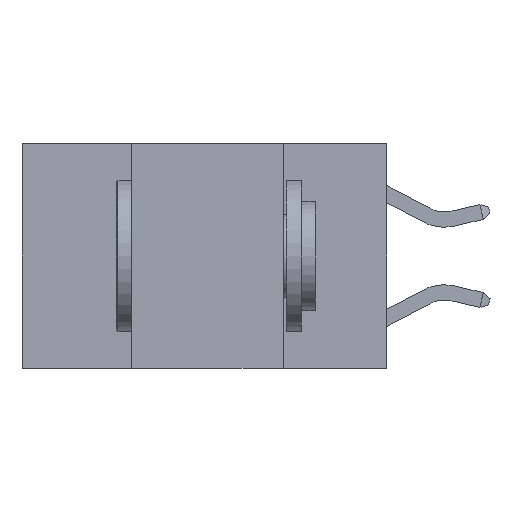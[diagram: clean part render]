
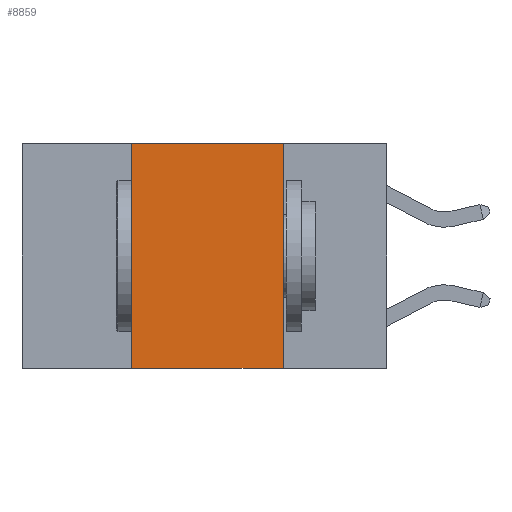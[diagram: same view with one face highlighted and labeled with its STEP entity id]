
A CAD part, left-side view. The second image highlights one B-rep face of the part: STEP entity #8859.
In plain terms, the highlighted planar face has unit normal (-1, 0, 0).
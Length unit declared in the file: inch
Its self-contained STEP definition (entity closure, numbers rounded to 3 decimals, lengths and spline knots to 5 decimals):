
#176 = VERTEX_POINT ( 'NONE', #12763 ) ;
#252 = PLANE ( 'NONE',  #11860 ) ;
#392 = CARTESIAN_POINT ( 'NONE',  ( 0., 0.6, 0. ) ) ;
#2381 = EDGE_CURVE ( 'NONE', #11145, #176, #7924, .T. ) ;
#2839 = FACE_OUTER_BOUND ( 'NONE', #3261, .T. ) ;
#3261 = EDGE_LOOP ( 'NONE', ( #10257, #10424, #11342, #3564 ) ) ;
#3564 = ORIENTED_EDGE ( 'NONE', *, *, #5597, .T. ) ;
#3608 = VERTEX_POINT ( 'NONE', #7484 ) ;
#3792 = VERTEX_POINT ( 'NONE', #4739 ) ;
#4494 = LINE ( 'NONE', #392, #9516 ) ;
#4739 = CARTESIAN_POINT ( 'NONE',  ( 0., 0.17, 0. ) ) ;
#5171 = CARTESIAN_POINT ( 'NONE',  ( 0., 0.17, 0. ) ) ;
#5269 = DIRECTION ( 'NONE',  ( 0., 0., -1. ) ) ;
#5597 = EDGE_CURVE ( 'NONE', #11145, #3608, #9882, .T. ) ;
#5792 = VECTOR ( 'NONE', #7195, 39.37008 ) ;
#5926 = EDGE_CURVE ( 'NONE', #3792, #3608, #8476, .T. ) ;
#6705 = CARTESIAN_POINT ( 'NONE',  ( 0., 0.6, -0.37 ) ) ;
#7195 = DIRECTION ( 'NONE',  ( 0., 0., -1. ) ) ;
#7484 = CARTESIAN_POINT ( 'NONE',  ( 0., 0.17, -0.37 ) ) ;
#7616 = VECTOR ( 'NONE', #11719, 39.37008 ) ;
#7924 = LINE ( 'NONE', #9748, #7616 ) ;
#8218 = CARTESIAN_POINT ( 'NONE',  ( 0., 0.6, 0. ) ) ;
#8476 = LINE ( 'NONE', #5171, #5792 ) ;
#8859 = ADVANCED_FACE ( 'NONE', ( #2839 ), #252, .F. ) ;
#9516 = VECTOR ( 'NONE', #12308, 39.37008 ) ;
#9748 = CARTESIAN_POINT ( 'NONE',  ( 0., 0.42, 0. ) ) ;
#9882 = LINE ( 'NONE', #6705, #12809 ) ;
#9948 = CARTESIAN_POINT ( 'NONE',  ( 0., 0.42, -0.37 ) ) ;
#10257 = ORIENTED_EDGE ( 'NONE', *, *, #5926, .F. ) ;
#10424 = ORIENTED_EDGE ( 'NONE', *, *, #10774, .F. ) ;
#10677 = DIRECTION ( 'NONE',  ( 0., -1., 0. ) ) ;
#10774 = EDGE_CURVE ( 'NONE', #176, #3792, #4494, .T. ) ;
#11145 = VERTEX_POINT ( 'NONE', #9948 ) ;
#11241 = DIRECTION ( 'NONE',  ( 1., 0., 0. ) ) ;
#11342 = ORIENTED_EDGE ( 'NONE', *, *, #2381, .F. ) ;
#11719 = DIRECTION ( 'NONE',  ( 0., 0., 1. ) ) ;
#11860 = AXIS2_PLACEMENT_3D ( 'NONE', #8218, #11241, #5269 ) ;
#12308 = DIRECTION ( 'NONE',  ( 0., -1., 0. ) ) ;
#12763 = CARTESIAN_POINT ( 'NONE',  ( 0., 0.42, 0. ) ) ;
#12809 = VECTOR ( 'NONE', #10677, 39.37008 ) ;
